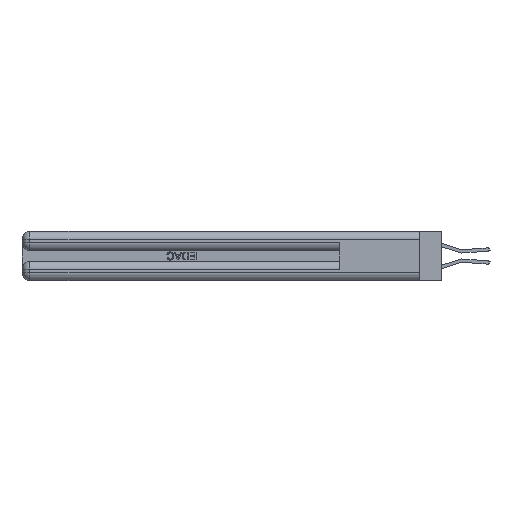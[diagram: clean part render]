
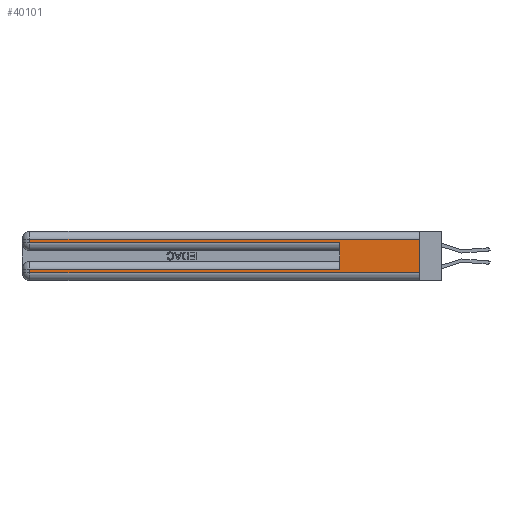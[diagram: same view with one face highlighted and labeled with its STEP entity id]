
A CAD part, left-side view. The second image highlights one B-rep face of the part: STEP entity #40101.
In plain terms, the highlighted planar face has unit normal (-1, 0, 0).
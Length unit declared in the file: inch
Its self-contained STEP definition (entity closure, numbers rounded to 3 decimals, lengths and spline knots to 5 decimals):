
#381 = VECTOR ( 'NONE', #29252, 39.37008 ) ;
#572 = DIRECTION ( 'NONE',  ( 0., 0., -1. ) ) ;
#582 = ORIENTED_EDGE ( 'NONE', *, *, #30322, .F. ) ;
#1823 = EDGE_CURVE ( 'NONE', #23727, #22195, #33141, .T. ) ;
#2283 = LINE ( 'NONE', #24685, #33953 ) ;
#2302 = VERTEX_POINT ( 'NONE', #28943 ) ;
#2396 = VERTEX_POINT ( 'NONE', #26108 ) ;
#2564 = ORIENTED_EDGE ( 'NONE', *, *, #7808, .F. ) ;
#2705 = DIRECTION ( 'NONE',  ( 0., 0., -1. ) ) ;
#3305 = VERTEX_POINT ( 'NONE', #35392 ) ;
#3372 = LINE ( 'NONE', #14298, #381 ) ;
#3482 = VECTOR ( 'NONE', #31381, 39.37008 ) ;
#4207 = EDGE_CURVE ( 'NONE', #2302, #31643, #15993, .T. ) ;
#4222 = ORIENTED_EDGE ( 'NONE', *, *, #1823, .T. ) ;
#5762 = CARTESIAN_POINT ( 'NONE',  ( 0., 2.94, 0.31 ) ) ;
#6447 = CARTESIAN_POINT ( 'NONE',  ( 0., 0., 0.085 ) ) ;
#7808 = EDGE_CURVE ( 'NONE', #2396, #3305, #23056, .T. ) ;
#8281 = EDGE_CURVE ( 'NONE', #22436, #2302, #23983, .T. ) ;
#8661 = ORIENTED_EDGE ( 'NONE', *, *, #23343, .T. ) ;
#9281 = VECTOR ( 'NONE', #36331, 39.37008 ) ;
#9687 = EDGE_LOOP ( 'NONE', ( #2564, #13931, #8661, #4222, #582, #27711, #10577, #15763 ) ) ;
#9776 = VECTOR ( 'NONE', #18508, 39.37008 ) ;
#9983 = CARTESIAN_POINT ( 'NONE',  ( 0., 0.6, 0.085 ) ) ;
#10577 = ORIENTED_EDGE ( 'NONE', *, *, #4207, .T. ) ;
#12224 = LINE ( 'NONE', #14948, #9776 ) ;
#12305 = CARTESIAN_POINT ( 'NONE',  ( 0., 0.6, 0.285 ) ) ;
#13470 = FACE_OUTER_BOUND ( 'NONE', #9687, .T. ) ;
#13931 = ORIENTED_EDGE ( 'NONE', *, *, #21561, .T. ) ;
#14298 = CARTESIAN_POINT ( 'NONE',  ( 0., 0.6, 0.145 ) ) ;
#14948 = CARTESIAN_POINT ( 'NONE',  ( 0., 0., 0.31 ) ) ;
#15147 = DIRECTION ( 'NONE',  ( 0., -1., 0. ) ) ;
#15763 = ORIENTED_EDGE ( 'NONE', *, *, #31801, .T. ) ;
#15814 = CARTESIAN_POINT ( 'NONE',  ( 0., 2.94, 0.37 ) ) ;
#15993 = LINE ( 'NONE', #15814, #39870 ) ;
#18508 = DIRECTION ( 'NONE',  ( 0., 1., 0. ) ) ;
#19241 = DIRECTION ( 'NONE',  ( 0., 0., -1. ) ) ;
#20131 = VECTOR ( 'NONE', #572, 39.37008 ) ;
#21502 = LINE ( 'NONE', #30062, #39461 ) ;
#21561 = EDGE_CURVE ( 'NONE', #2396, #22320, #12224, .T. ) ;
#22195 = VERTEX_POINT ( 'NONE', #12305 ) ;
#22229 = PLANE ( 'NONE',  #27784 ) ;
#22320 = VERTEX_POINT ( 'NONE', #5762 ) ;
#22436 = VERTEX_POINT ( 'NONE', #9983 ) ;
#23056 = LINE ( 'NONE', #25269, #20131 ) ;
#23343 = EDGE_CURVE ( 'NONE', #22320, #23727, #21502, .T. ) ;
#23727 = VERTEX_POINT ( 'NONE', #26846 ) ;
#23983 = LINE ( 'NONE', #6447, #3482 ) ;
#24685 = CARTESIAN_POINT ( 'NONE',  ( 0., 0., 0.06 ) ) ;
#25269 = CARTESIAN_POINT ( 'NONE',  ( 0., 0., 0.37 ) ) ;
#26108 = CARTESIAN_POINT ( 'NONE',  ( 0., 0., 0.31 ) ) ;
#26846 = CARTESIAN_POINT ( 'NONE',  ( 0., 2.94, 0.285 ) ) ;
#27711 = ORIENTED_EDGE ( 'NONE', *, *, #8281, .T. ) ;
#27784 = AXIS2_PLACEMENT_3D ( 'NONE', #34834, #31324, #28183 ) ;
#28183 = DIRECTION ( 'NONE',  ( 0., 0., -1. ) ) ;
#28943 = CARTESIAN_POINT ( 'NONE',  ( 0., 2.94, 0.085 ) ) ;
#29252 = DIRECTION ( 'NONE',  ( 0., 0., 1. ) ) ;
#30062 = CARTESIAN_POINT ( 'NONE',  ( 0., 2.94, 0.37 ) ) ;
#30322 = EDGE_CURVE ( 'NONE', #22436, #22195, #3372, .T. ) ;
#31324 = DIRECTION ( 'NONE',  ( 1., 0., 0. ) ) ;
#31381 = DIRECTION ( 'NONE',  ( 0., 1., 0. ) ) ;
#31643 = VERTEX_POINT ( 'NONE', #39387 ) ;
#31801 = EDGE_CURVE ( 'NONE', #31643, #3305, #2283, .T. ) ;
#33141 = LINE ( 'NONE', #33224, #9281 ) ;
#33224 = CARTESIAN_POINT ( 'NONE',  ( 0., 0., 0.285 ) ) ;
#33953 = VECTOR ( 'NONE', #15147, 39.37008 ) ;
#34834 = CARTESIAN_POINT ( 'NONE',  ( 0., 0., 0.37 ) ) ;
#35392 = CARTESIAN_POINT ( 'NONE',  ( 0., 0., 0.06 ) ) ;
#36331 = DIRECTION ( 'NONE',  ( 0., -1., 0. ) ) ;
#39387 = CARTESIAN_POINT ( 'NONE',  ( 0., 2.94, 0.06 ) ) ;
#39461 = VECTOR ( 'NONE', #2705, 39.37008 ) ;
#39870 = VECTOR ( 'NONE', #19241, 39.37008 ) ;
#40101 = ADVANCED_FACE ( 'NONE', ( #13470 ), #22229, .F. ) ;
